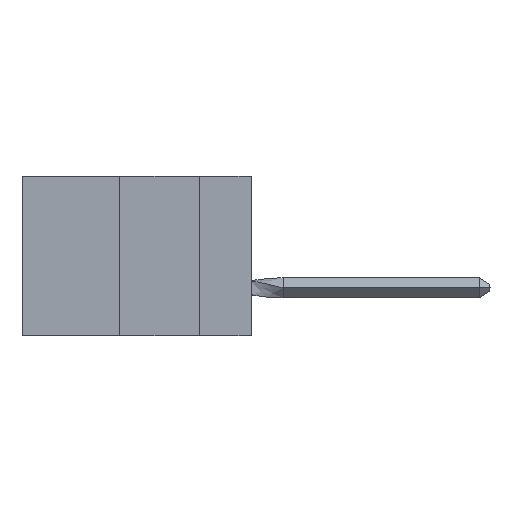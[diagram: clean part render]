
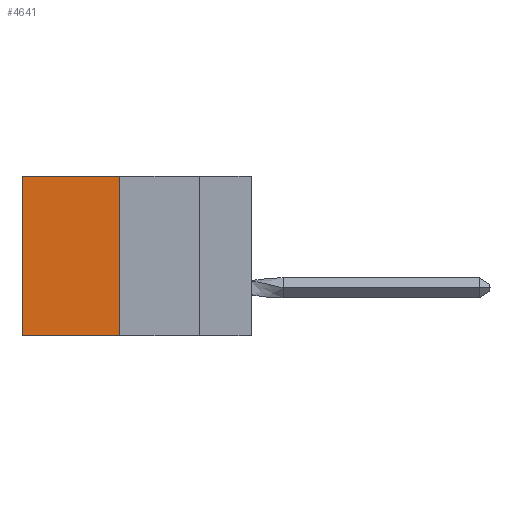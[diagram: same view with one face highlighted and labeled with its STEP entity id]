
A CAD part, left-side view. The second image highlights one B-rep face of the part: STEP entity #4641.
In plain terms, the highlighted planar face has unit normal (-1, 0, 0).
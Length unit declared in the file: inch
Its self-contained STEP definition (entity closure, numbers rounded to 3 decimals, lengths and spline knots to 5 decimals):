
#671 = LINE ( 'NONE', #8517, #9918 ) ;
#792 = FACE_OUTER_BOUND ( 'NONE', #5943, .T. ) ;
#1304 = CARTESIAN_POINT ( 'NONE',  ( 0.305, 0.413, -0.5 ) ) ;
#1341 = CARTESIAN_POINT ( 'NONE',  ( 0.305, 0.413, -0.5 ) ) ;
#2081 = CARTESIAN_POINT ( 'NONE',  ( 0.305, 0.413, -0.5 ) ) ;
#2425 = VERTEX_POINT ( 'NONE', #1341 ) ;
#2707 = LINE ( 'NONE', #2081, #7187 ) ;
#2979 = EDGE_CURVE ( 'NONE', #2425, #6001, #671, .T. ) ;
#3673 = CARTESIAN_POINT ( 'NONE',  ( 0.305, 0.72, 0. ) ) ;
#3888 = VERTEX_POINT ( 'NONE', #13180 ) ;
#4261 = ORIENTED_EDGE ( 'NONE', *, *, #13603, .T. ) ;
#4298 = CARTESIAN_POINT ( 'NONE',  ( 0.305, 0.72, -0.5 ) ) ;
#4373 = DIRECTION ( 'NONE',  ( 0., 1., 0. ) ) ;
#4374 = AXIS2_PLACEMENT_3D ( 'NONE', #1304, #8584, #12936 ) ;
#4641 = ADVANCED_FACE ( 'NONE', ( #792 ), #7474, .F. ) ;
#5363 = ORIENTED_EDGE ( 'NONE', *, *, #10292, .F. ) ;
#5619 = DIRECTION ( 'NONE',  ( 0., 1., 0. ) ) ;
#5943 = EDGE_LOOP ( 'NONE', ( #4261, #6889, #5363, #11998 ) ) ;
#6001 = VERTEX_POINT ( 'NONE', #4298 ) ;
#6385 = DIRECTION ( 'NONE',  ( 0., 0., -1. ) ) ;
#6889 = ORIENTED_EDGE ( 'NONE', *, *, #2979, .F. ) ;
#7187 = VECTOR ( 'NONE', #6385, 39.37008 ) ;
#7474 = PLANE ( 'NONE',  #4374 ) ;
#7667 = LINE ( 'NONE', #8732, #13012 ) ;
#8059 = VECTOR ( 'NONE', #12300, 39.37008 ) ;
#8517 = CARTESIAN_POINT ( 'NONE',  ( 0.305, 0.413, -0.5 ) ) ;
#8584 = DIRECTION ( 'NONE',  ( 1., 0., 0. ) ) ;
#8732 = CARTESIAN_POINT ( 'NONE',  ( 0.305, 0.413, 0. ) ) ;
#9918 = VECTOR ( 'NONE', #4373, 39.37008 ) ;
#10292 = EDGE_CURVE ( 'NONE', #3888, #2425, #2707, .T. ) ;
#10339 = CARTESIAN_POINT ( 'NONE',  ( 0.305, 0.72, -0.5 ) ) ;
#10371 = EDGE_CURVE ( 'NONE', #3888, #11195, #7667, .T. ) ;
#11195 = VERTEX_POINT ( 'NONE', #3673 ) ;
#11998 = ORIENTED_EDGE ( 'NONE', *, *, #10371, .T. ) ;
#12300 = DIRECTION ( 'NONE',  ( 0., 0., -1. ) ) ;
#12591 = LINE ( 'NONE', #10339, #8059 ) ;
#12936 = DIRECTION ( 'NONE',  ( 0., 0., -1. ) ) ;
#13012 = VECTOR ( 'NONE', #5619, 39.37008 ) ;
#13180 = CARTESIAN_POINT ( 'NONE',  ( 0.305, 0.413, 0. ) ) ;
#13603 = EDGE_CURVE ( 'NONE', #11195, #6001, #12591, .T. ) ;
